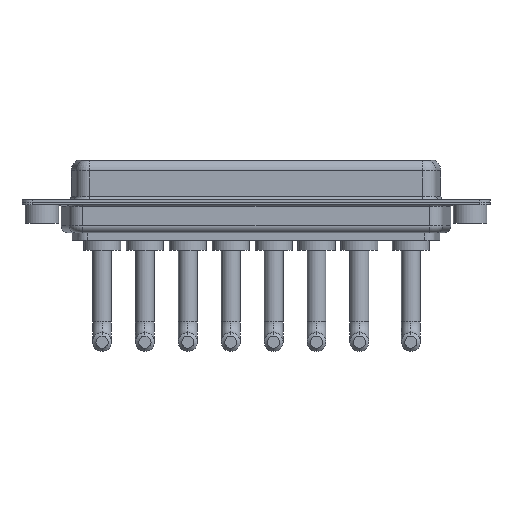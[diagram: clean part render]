
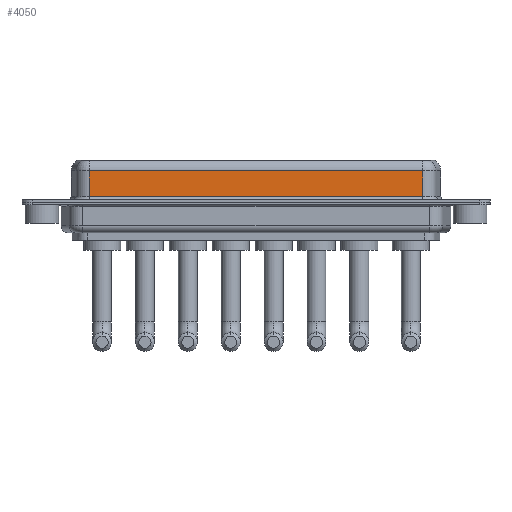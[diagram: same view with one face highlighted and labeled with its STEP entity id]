
A CAD part, front view. The second image highlights one B-rep face of the part: STEP entity #4050.
In plain terms, the highlighted planar face has unit normal (0, -1, 0).
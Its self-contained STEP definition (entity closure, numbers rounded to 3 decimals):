
#447 = DIRECTION ( 'NONE',  ( 0., 0., 1. ) ) ;
#470 = CARTESIAN_POINT ( 'NONE',  ( 7.038, -3.95, 0.9 ) ) ;
#523 = VERTEX_POINT ( 'NONE', #9053 ) ;
#777 = EDGE_LOOP ( 'NONE', ( #10435, #4930, #10088, #6436 ) ) ;
#1376 = FACE_OUTER_BOUND ( 'NONE', #777, .T. ) ;
#1878 = EDGE_CURVE ( 'NONE', #7978, #5661, #8996, .T. ) ;
#3293 = EDGE_CURVE ( 'NONE', #5075, #5661, #6274, .T. ) ;
#3824 = VECTOR ( 'NONE', #5019, 1000. ) ;
#4050 = ADVANCED_FACE ( 'NONE', ( #1376 ), #8537, .F. ) ;
#4776 = CARTESIAN_POINT ( 'NONE',  ( 56.462, -3.95, 4.65 ) ) ;
#4930 = ORIENTED_EDGE ( 'NONE', *, *, #9974, .T. ) ;
#5019 = DIRECTION ( 'NONE',  ( 0., 0., -1. ) ) ;
#5075 = VERTEX_POINT ( 'NONE', #470 ) ;
#5535 = CARTESIAN_POINT ( 'NONE',  ( 56.462, -3.95, 6.4 ) ) ;
#5661 = VERTEX_POINT ( 'NONE', #8669 ) ;
#5909 = CARTESIAN_POINT ( 'NONE',  ( 56.462, -3.95, 6.4 ) ) ;
#6274 = LINE ( 'NONE', #11289, #7344 ) ;
#6436 = ORIENTED_EDGE ( 'NONE', *, *, #3293, .T. ) ;
#6982 = LINE ( 'NONE', #4776, #8333 ) ;
#7228 = CARTESIAN_POINT ( 'NONE',  ( 7.038, -3.95, 6.4 ) ) ;
#7344 = VECTOR ( 'NONE', #13242, 1000. ) ;
#7519 = VECTOR ( 'NONE', #9115, 1000. ) ;
#7978 = VERTEX_POINT ( 'NONE', #8393 ) ;
#8333 = VECTOR ( 'NONE', #10131, 1000. ) ;
#8393 = CARTESIAN_POINT ( 'NONE',  ( 56.462, -3.95, 4.65 ) ) ;
#8537 = PLANE ( 'NONE',  #9887 ) ;
#8669 = CARTESIAN_POINT ( 'NONE',  ( 56.462, -3.95, 0.9 ) ) ;
#8996 = LINE ( 'NONE', #5909, #7519 ) ;
#9053 = CARTESIAN_POINT ( 'NONE',  ( 7.038, -3.95, 4.65 ) ) ;
#9115 = DIRECTION ( 'NONE',  ( 0., 0., -1. ) ) ;
#9602 = DIRECTION ( 'NONE',  ( 0., 1., 0. ) ) ;
#9887 = AXIS2_PLACEMENT_3D ( 'NONE', #5535, #9602, #447 ) ;
#9974 = EDGE_CURVE ( 'NONE', #7978, #523, #6982, .T. ) ;
#10088 = ORIENTED_EDGE ( 'NONE', *, *, #12198, .T. ) ;
#10131 = DIRECTION ( 'NONE',  ( -1., 0., 0. ) ) ;
#10435 = ORIENTED_EDGE ( 'NONE', *, *, #1878, .F. ) ;
#11289 = CARTESIAN_POINT ( 'NONE',  ( 56.462, -3.95, 0.9 ) ) ;
#12198 = EDGE_CURVE ( 'NONE', #523, #5075, #12331, .T. ) ;
#12331 = LINE ( 'NONE', #7228, #3824 ) ;
#13242 = DIRECTION ( 'NONE',  ( 1., 0., 0. ) ) ;
